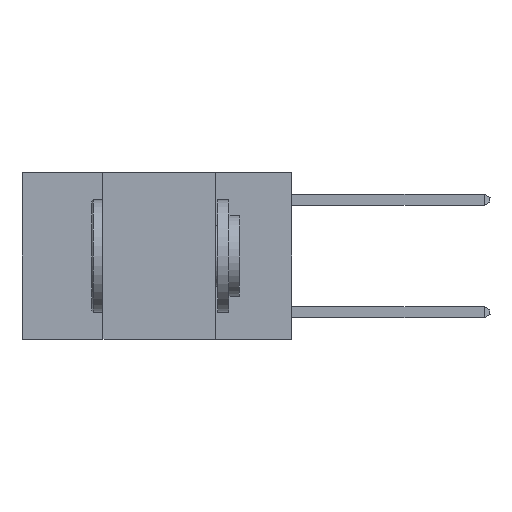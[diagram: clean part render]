
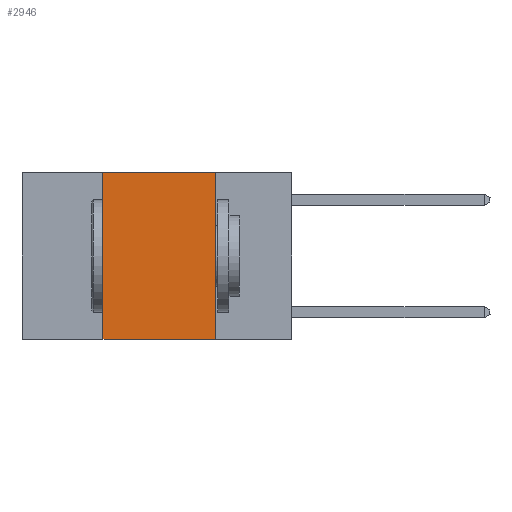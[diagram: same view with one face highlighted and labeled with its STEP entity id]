
A CAD part, left-side view. The second image highlights one B-rep face of the part: STEP entity #2946.
In plain terms, the highlighted planar face has unit normal (-1, 0, 0).
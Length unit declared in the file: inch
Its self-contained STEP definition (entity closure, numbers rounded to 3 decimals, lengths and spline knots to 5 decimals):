
#98 = DIRECTION ( 'NONE',  ( 0., 0., -1. ) ) ;
#446 = LINE ( 'NONE', #9365, #8531 ) ;
#871 = PLANE ( 'NONE',  #10254 ) ;
#1000 = VERTEX_POINT ( 'NONE', #5343 ) ;
#1021 = CARTESIAN_POINT ( 'NONE',  ( 0., 0.6, 0. ) ) ;
#1650 = EDGE_CURVE ( 'NONE', #4282, #1000, #4625, .T. ) ;
#1708 = FACE_OUTER_BOUND ( 'NONE', #5436, .T. ) ;
#1806 = VERTEX_POINT ( 'NONE', #3410 ) ;
#2450 = LINE ( 'NONE', #4766, #2816 ) ;
#2816 = VECTOR ( 'NONE', #4065, 39.37008 ) ;
#2946 = ADVANCED_FACE ( 'NONE', ( #1708 ), #871, .F. ) ;
#3410 = CARTESIAN_POINT ( 'NONE',  ( 0., 0.42, 0. ) ) ;
#4065 = DIRECTION ( 'NONE',  ( 0., 0., 1. ) ) ;
#4282 = VERTEX_POINT ( 'NONE', #10399 ) ;
#4289 = DIRECTION ( 'NONE',  ( 1., 0., 0. ) ) ;
#4625 = LINE ( 'NONE', #8024, #5526 ) ;
#4766 = CARTESIAN_POINT ( 'NONE',  ( 0., 0.42, 0. ) ) ;
#5343 = CARTESIAN_POINT ( 'NONE',  ( 0., 0.17, -0.37 ) ) ;
#5436 = EDGE_LOOP ( 'NONE', ( #8117, #5777, #6987, #9955 ) ) ;
#5502 = EDGE_CURVE ( 'NONE', #1806, #6716, #446, .T. ) ;
#5526 = VECTOR ( 'NONE', #7859, 39.37008 ) ;
#5777 = ORIENTED_EDGE ( 'NONE', *, *, #5502, .F. ) ;
#5811 = LINE ( 'NONE', #9791, #8924 ) ;
#6716 = VERTEX_POINT ( 'NONE', #7429 ) ;
#6987 = ORIENTED_EDGE ( 'NONE', *, *, #7010, .F. ) ;
#7010 = EDGE_CURVE ( 'NONE', #4282, #1806, #2450, .T. ) ;
#7429 = CARTESIAN_POINT ( 'NONE',  ( 0., 0.17, 0. ) ) ;
#7780 = DIRECTION ( 'NONE',  ( 0., -1., 0. ) ) ;
#7859 = DIRECTION ( 'NONE',  ( 0., -1., 0. ) ) ;
#7876 = EDGE_CURVE ( 'NONE', #6716, #1000, #5811, .T. ) ;
#8024 = CARTESIAN_POINT ( 'NONE',  ( 0., 0.6, -0.37 ) ) ;
#8117 = ORIENTED_EDGE ( 'NONE', *, *, #7876, .F. ) ;
#8531 = VECTOR ( 'NONE', #7780, 39.37008 ) ;
#8924 = VECTOR ( 'NONE', #8986, 39.37008 ) ;
#8986 = DIRECTION ( 'NONE',  ( 0., 0., -1. ) ) ;
#9365 = CARTESIAN_POINT ( 'NONE',  ( 0., 0.6, 0. ) ) ;
#9791 = CARTESIAN_POINT ( 'NONE',  ( 0., 0.17, 0. ) ) ;
#9955 = ORIENTED_EDGE ( 'NONE', *, *, #1650, .T. ) ;
#10254 = AXIS2_PLACEMENT_3D ( 'NONE', #1021, #4289, #98 ) ;
#10399 = CARTESIAN_POINT ( 'NONE',  ( 0., 0.42, -0.37 ) ) ;
